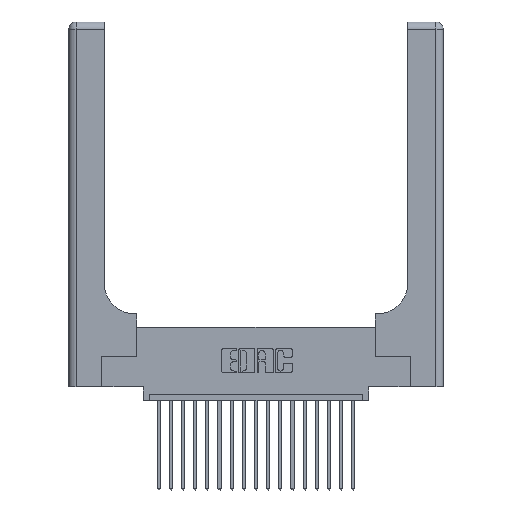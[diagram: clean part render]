
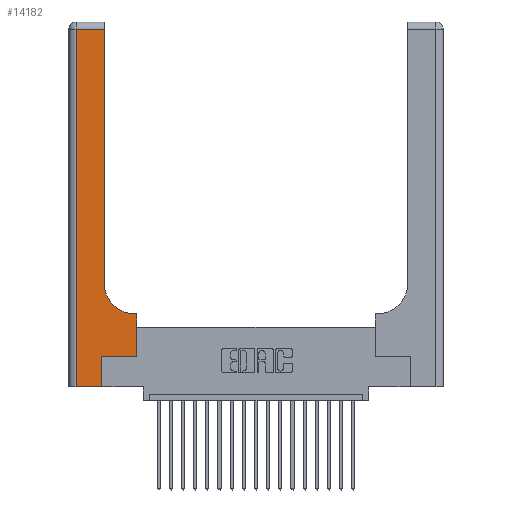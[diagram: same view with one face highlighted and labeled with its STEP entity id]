
A CAD part, top view. The second image highlights one B-rep face of the part: STEP entity #14182.
In plain terms, the highlighted planar face has unit normal (0, 0, 1).
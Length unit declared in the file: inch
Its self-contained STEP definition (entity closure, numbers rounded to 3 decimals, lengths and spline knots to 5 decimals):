
#7 = CARTESIAN_POINT ( 'NONE',  ( 0., 0., 0.37 ) ) ;
#409 = CARTESIAN_POINT ( 'NONE',  ( 0.06, 3., 0.37 ) ) ;
#1095 = DIRECTION ( 'NONE',  ( 0., 1., 0. ) ) ;
#1203 = VERTEX_POINT ( 'NONE', #8376 ) ;
#1340 = VERTEX_POINT ( 'NONE', #18883 ) ;
#1426 = DIRECTION ( 'NONE',  ( 0., 1., 0. ) ) ;
#1685 = DIRECTION ( 'NONE',  ( 1., 0., 0. ) ) ;
#1780 = DIRECTION ( 'NONE',  ( 1., 0., 0. ) ) ;
#1902 = VECTOR ( 'NONE', #3663, 39.37008 ) ;
#2010 = DIRECTION ( 'NONE',  ( 0., -1., 0. ) ) ;
#2014 = VECTOR ( 'NONE', #14104, 39.37008 ) ;
#2227 = CARTESIAN_POINT ( 'NONE',  ( 0., 3., 0.37 ) ) ;
#2638 = EDGE_CURVE ( 'NONE', #1340, #9453, #16033, .T. ) ;
#2686 = CARTESIAN_POINT ( 'NONE',  ( 0.2915, 2.94, 0.37 ) ) ;
#2855 = EDGE_CURVE ( 'NONE', #13195, #7958, #6169, .T. ) ;
#3113 = CARTESIAN_POINT ( 'NONE',  ( 0.2915, 0.85, 0.37 ) ) ;
#3343 = VECTOR ( 'NONE', #1685, 39.37008 ) ;
#3477 = CARTESIAN_POINT ( 'NONE',  ( 0.2915, 3., 0.37 ) ) ;
#3663 = DIRECTION ( 'NONE',  ( -1., 0., 0. ) ) ;
#4155 = CARTESIAN_POINT ( 'NONE',  ( 0.5585, 0.25, 0.37 ) ) ;
#4360 = CARTESIAN_POINT ( 'NONE',  ( 0.2915, 0.6, 0.37 ) ) ;
#5780 = EDGE_CURVE ( 'NONE', #1203, #13883, #20827, .T. ) ;
#6169 = LINE ( 'NONE', #7, #3343 ) ;
#7302 = DIRECTION ( 'NONE',  ( 0., 0., -1. ) ) ;
#7958 = VERTEX_POINT ( 'NONE', #8014 ) ;
#8014 = CARTESIAN_POINT ( 'NONE',  ( 0.269, 0., 0.37 ) ) ;
#8051 = ORIENTED_EDGE ( 'NONE', *, *, #2855, .T. ) ;
#8376 = CARTESIAN_POINT ( 'NONE',  ( 0.5415, 0.6, 0.37 ) ) ;
#8420 = LINE ( 'NONE', #18808, #1902 ) ;
#8619 = VECTOR ( 'NONE', #2010, 39.37008 ) ;
#8771 = PLANE ( 'NONE',  #19916 ) ;
#8875 = VECTOR ( 'NONE', #1095, 39.37008 ) ;
#9236 = CARTESIAN_POINT ( 'NONE',  ( 0.06, 0., 0.37 ) ) ;
#9453 = VERTEX_POINT ( 'NONE', #17240 ) ;
#9967 = AXIS2_PLACEMENT_3D ( 'NONE', #20063, #13456, #1780 ) ;
#10036 = VERTEX_POINT ( 'NONE', #2686 ) ;
#10310 = VECTOR ( 'NONE', #1426, 39.37008 ) ;
#10368 = DIRECTION ( 'NONE',  ( 0., 1., 0. ) ) ;
#10891 = ORIENTED_EDGE ( 'NONE', *, *, #19124, .T. ) ;
#11281 = CARTESIAN_POINT ( 'NONE',  ( 0.269, 0., 0.37 ) ) ;
#11537 = EDGE_CURVE ( 'NONE', #7958, #1340, #14696, .T. ) ;
#11545 = EDGE_LOOP ( 'NONE', ( #19060, #16096, #10891, #8051, #11841, #14500, #16742, #20933, #19937 ) ) ;
#11841 = ORIENTED_EDGE ( 'NONE', *, *, #11537, .T. ) ;
#12405 = EDGE_CURVE ( 'NONE', #17874, #1203, #18044, .T. ) ;
#12516 = FACE_OUTER_BOUND ( 'NONE', #11545, .T. ) ;
#13195 = VERTEX_POINT ( 'NONE', #9236 ) ;
#13413 = CARTESIAN_POINT ( 'NONE',  ( 0.5585, 0.6, 0.37 ) ) ;
#13456 = DIRECTION ( 'NONE',  ( 0., 0., -1. ) ) ;
#13740 = CARTESIAN_POINT ( 'NONE',  ( 0.269, 0.25, 0.37 ) ) ;
#13883 = VERTEX_POINT ( 'NONE', #3113 ) ;
#14028 = EDGE_CURVE ( 'NONE', #13883, #10036, #21077, .T. ) ;
#14104 = DIRECTION ( 'NONE',  ( 1., 0., 0. ) ) ;
#14160 = DIRECTION ( 'NONE',  ( -1., 0., 0. ) ) ;
#14182 = ADVANCED_FACE ( 'NONE', ( #12516 ), #8771, .F. ) ;
#14500 = ORIENTED_EDGE ( 'NONE', *, *, #2638, .T. ) ;
#14696 = LINE ( 'NONE', #11281, #10310 ) ;
#16033 = LINE ( 'NONE', #13740, #2014 ) ;
#16096 = ORIENTED_EDGE ( 'NONE', *, *, #17179, .T. ) ;
#16384 = VERTEX_POINT ( 'NONE', #16644 ) ;
#16644 = CARTESIAN_POINT ( 'NONE',  ( 0.06, 2.94, 0.37 ) ) ;
#16742 = ORIENTED_EDGE ( 'NONE', *, *, #18770, .T. ) ;
#16998 = VECTOR ( 'NONE', #14160, 39.37008 ) ;
#17101 = DIRECTION ( 'NONE',  ( -1., 0., 0. ) ) ;
#17179 = EDGE_CURVE ( 'NONE', #10036, #16384, #8420, .T. ) ;
#17240 = CARTESIAN_POINT ( 'NONE',  ( 0.5585, 0.25, 0.37 ) ) ;
#17716 = VECTOR ( 'NONE', #10368, 39.37008 ) ;
#17874 = VERTEX_POINT ( 'NONE', #13413 ) ;
#17935 = LINE ( 'NONE', #4155, #8875 ) ;
#18044 = LINE ( 'NONE', #4360, #16998 ) ;
#18770 = EDGE_CURVE ( 'NONE', #9453, #17874, #17935, .T. ) ;
#18808 = CARTESIAN_POINT ( 'NONE',  ( 0., 2.94, 0.37 ) ) ;
#18883 = CARTESIAN_POINT ( 'NONE',  ( 0.269, 0.25, 0.37 ) ) ;
#19060 = ORIENTED_EDGE ( 'NONE', *, *, #14028, .T. ) ;
#19124 = EDGE_CURVE ( 'NONE', #16384, #13195, #19222, .T. ) ;
#19222 = LINE ( 'NONE', #409, #8619 ) ;
#19916 = AXIS2_PLACEMENT_3D ( 'NONE', #2227, #7302, #17101 ) ;
#19937 = ORIENTED_EDGE ( 'NONE', *, *, #5780, .T. ) ;
#20063 = CARTESIAN_POINT ( 'NONE',  ( 0.5415, 0.85, 0.37 ) ) ;
#20827 = CIRCLE ( 'NONE', #9967, 0.25 ) ;
#20933 = ORIENTED_EDGE ( 'NONE', *, *, #12405, .T. ) ;
#21077 = LINE ( 'NONE', #3477, #17716 ) ;
